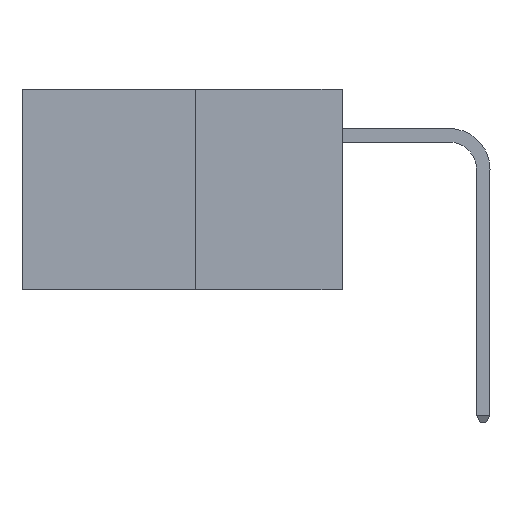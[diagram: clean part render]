
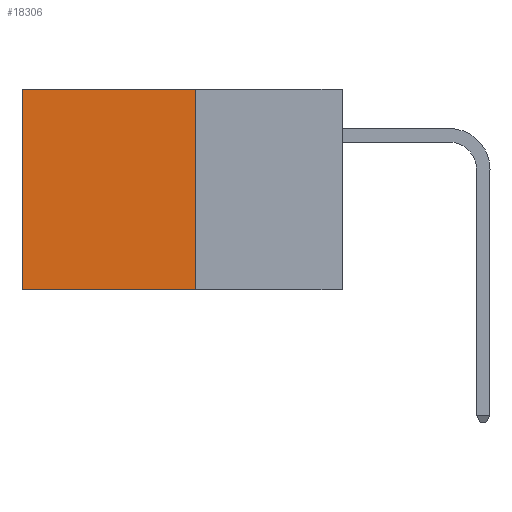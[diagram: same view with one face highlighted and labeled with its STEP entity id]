
A CAD part, left-side view. The second image highlights one B-rep face of the part: STEP entity #18306.
In plain terms, the highlighted planar face has unit normal (-1, 0, 0).
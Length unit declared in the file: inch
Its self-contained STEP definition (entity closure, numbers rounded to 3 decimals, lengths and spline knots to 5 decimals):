
#1721 = EDGE_CURVE ( 'NONE', #23855, #9021, #10508, .T. ) ;
#1802 = EDGE_CURVE ( 'NONE', #9650, #9021, #27010, .T. ) ;
#1884 = CARTESIAN_POINT ( 'NONE',  ( 0.277, 0.27, -0.37 ) ) ;
#1901 = DIRECTION ( 'NONE',  ( 0., 0., -1. ) ) ;
#3079 = VECTOR ( 'NONE', #15467, 39.37008 ) ;
#4517 = VECTOR ( 'NONE', #15575, 39.37008 ) ;
#4534 = CARTESIAN_POINT ( 'NONE',  ( 0.277, 0.27, -0.37 ) ) ;
#4668 = ORIENTED_EDGE ( 'NONE', *, *, #1721, .T. ) ;
#8382 = LINE ( 'NONE', #1884, #3079 ) ;
#9021 = VERTEX_POINT ( 'NONE', #10167 ) ;
#9650 = VERTEX_POINT ( 'NONE', #21259 ) ;
#10019 = ORIENTED_EDGE ( 'NONE', *, *, #11012, .T. ) ;
#10167 = CARTESIAN_POINT ( 'NONE',  ( 0.277, 0.59, -0.37 ) ) ;
#10508 = LINE ( 'NONE', #24499, #4517 ) ;
#10846 = CARTESIAN_POINT ( 'NONE',  ( 0.277, 0.27, -0.37 ) ) ;
#11012 = EDGE_CURVE ( 'NONE', #20716, #23855, #25864, .T. ) ;
#12193 = AXIS2_PLACEMENT_3D ( 'NONE', #10846, #15378, #1901 ) ;
#13127 = PLANE ( 'NONE',  #12193 ) ;
#15378 = DIRECTION ( 'NONE',  ( 1., 0., 0. ) ) ;
#15467 = DIRECTION ( 'NONE',  ( 0., 0., -1. ) ) ;
#15575 = DIRECTION ( 'NONE',  ( 0., 0., -1. ) ) ;
#18306 = ADVANCED_FACE ( 'NONE', ( #26949 ), #13127, .F. ) ;
#18487 = EDGE_LOOP ( 'NONE', ( #4668, #27480, #22586, #10019 ) ) ;
#19210 = VECTOR ( 'NONE', #25049, 39.37008 ) ;
#20716 = VERTEX_POINT ( 'NONE', #21612 ) ;
#21259 = CARTESIAN_POINT ( 'NONE',  ( 0.277, 0.27, -0.37 ) ) ;
#21612 = CARTESIAN_POINT ( 'NONE',  ( 0.277, 0.27, 0. ) ) ;
#22586 = ORIENTED_EDGE ( 'NONE', *, *, #25799, .F. ) ;
#23855 = VERTEX_POINT ( 'NONE', #28609 ) ;
#24499 = CARTESIAN_POINT ( 'NONE',  ( 0.277, 0.59, -0.37 ) ) ;
#25049 = DIRECTION ( 'NONE',  ( 0., 1., 0. ) ) ;
#25672 = CARTESIAN_POINT ( 'NONE',  ( 0.277, 0.27, 0. ) ) ;
#25799 = EDGE_CURVE ( 'NONE', #20716, #9650, #8382, .T. ) ;
#25864 = LINE ( 'NONE', #25672, #19210 ) ;
#26317 = VECTOR ( 'NONE', #27027, 39.37008 ) ;
#26949 = FACE_OUTER_BOUND ( 'NONE', #18487, .T. ) ;
#27010 = LINE ( 'NONE', #4534, #26317 ) ;
#27027 = DIRECTION ( 'NONE',  ( 0., 1., 0. ) ) ;
#27480 = ORIENTED_EDGE ( 'NONE', *, *, #1802, .F. ) ;
#28609 = CARTESIAN_POINT ( 'NONE',  ( 0.277, 0.59, 0. ) ) ;
